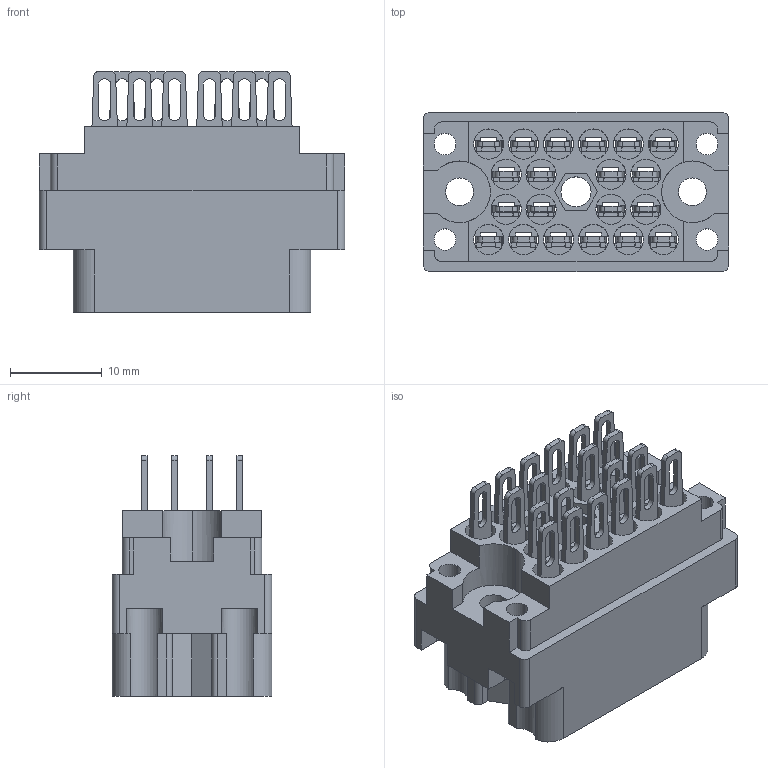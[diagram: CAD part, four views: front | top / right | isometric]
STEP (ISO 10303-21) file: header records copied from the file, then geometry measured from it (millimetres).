
FILE_DESCRIPTION (( 'STEP AP203' ), '1' );
FILE_NAME ('516-020-500-100.STEP', '2020-03-09T13:29:27', ( '' ), ( '' ), 'SwSTEP 2.0', 'SolidWorks 2016', '' );
FILE_SCHEMA (( 'CONFIG_CONTROL_DESIGN' ));
Length unit declared in the file: inch
Products named in the file (3): 516-020-500-100; 516 Plug Insulator_020; 516-292-001_500 Contact
Assembly tree (21 placements, depth 2):
  516-020-500-100
    516 Plug Insulator_020
    516-292-001_500 Contact  x20
Bounding box: 33.32 x 17.42 x 26.26 mm (x, y, z)
Volume: 5142.3 mm3; surface area: 10614.2 mm2
Topology: 21 solids, 21 shells, 2131 faces, 6193 edges, 4114 vertices
Faces by surface type: plane 1293, cylinder 716, bspline 120, cone 2
Entity records: 24015 total; most frequent: CARTESIAN_POINT 4349, ORIENTED_EDGE 4026, DIRECTION 3879, EDGE_CURVE 2013, LINE 1489, VECTOR 1489, VERTEX_POINT 1340, AXIS2_PLACEMENT_3D 1195
